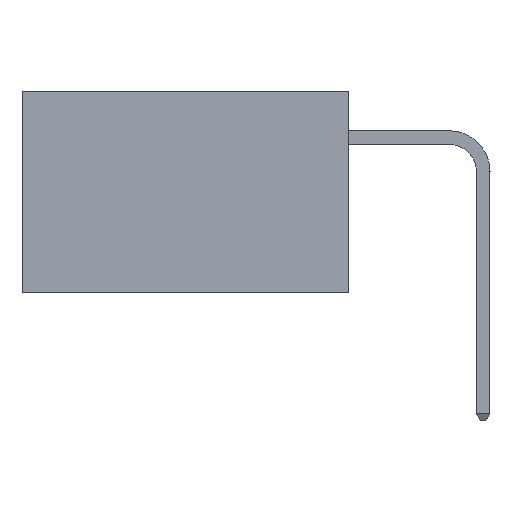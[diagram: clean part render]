
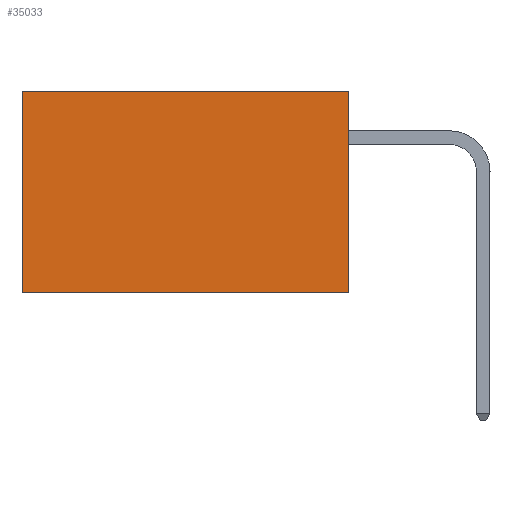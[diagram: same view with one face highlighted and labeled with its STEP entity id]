
A CAD part, left-side view. The second image highlights one B-rep face of the part: STEP entity #35033.
In plain terms, the highlighted planar face has unit normal (-1, 0, 0).
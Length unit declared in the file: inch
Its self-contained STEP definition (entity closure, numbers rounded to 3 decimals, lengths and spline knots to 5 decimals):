
#1095 = DIRECTION ( 'NONE',  ( 0., 1., 0. ) ) ;
#2598 = VERTEX_POINT ( 'NONE', #11360 ) ;
#3098 = CARTESIAN_POINT ( 'NONE',  ( 0.2875, 0., 0. ) ) ;
#3789 = CARTESIAN_POINT ( 'NONE',  ( 0.2875, 0., 0. ) ) ;
#5382 = VERTEX_POINT ( 'NONE', #20725 ) ;
#5522 = DIRECTION ( 'NONE',  ( 0., 0., -1. ) ) ;
#6307 = VERTEX_POINT ( 'NONE', #31010 ) ;
#6369 = ORIENTED_EDGE ( 'NONE', *, *, #20440, .F. ) ;
#6373 = DIRECTION ( 'NONE',  ( 0., 0., -1. ) ) ;
#7091 = EDGE_CURVE ( 'NONE', #6307, #5382, #21575, .T. ) ;
#8061 = LINE ( 'NONE', #3789, #22695 ) ;
#9188 = VECTOR ( 'NONE', #1095, 39.37008 ) ;
#11254 = DIRECTION ( 'NONE',  ( 0., 1., 0. ) ) ;
#11360 = CARTESIAN_POINT ( 'NONE',  ( 0.2875, 0.6, -0.37 ) ) ;
#11615 = EDGE_CURVE ( 'NONE', #14372, #2598, #17015, .T. ) ;
#14372 = VERTEX_POINT ( 'NONE', #28312 ) ;
#17015 = LINE ( 'NONE', #33896, #9188 ) ;
#17180 = CARTESIAN_POINT ( 'NONE',  ( 0.2875, 0., 0. ) ) ;
#18517 = ORIENTED_EDGE ( 'NONE', *, *, #35726, .T. ) ;
#18972 = LINE ( 'NONE', #23846, #35971 ) ;
#20125 = PLANE ( 'NONE',  #27266 ) ;
#20440 = EDGE_CURVE ( 'NONE', #6307, #14372, #8061, .T. ) ;
#20669 = VECTOR ( 'NONE', #11254, 39.37008 ) ;
#20725 = CARTESIAN_POINT ( 'NONE',  ( 0.2875, 0.6, 0. ) ) ;
#21575 = LINE ( 'NONE', #3098, #20669 ) ;
#22695 = VECTOR ( 'NONE', #35477, 39.37008 ) ;
#23015 = DIRECTION ( 'NONE',  ( 1., 0., 0. ) ) ;
#23846 = CARTESIAN_POINT ( 'NONE',  ( 0.2875, 0.6, 0. ) ) ;
#24268 = ORIENTED_EDGE ( 'NONE', *, *, #11615, .F. ) ;
#27266 = AXIS2_PLACEMENT_3D ( 'NONE', #17180, #23015, #5522 ) ;
#28312 = CARTESIAN_POINT ( 'NONE',  ( 0.2875, 0., -0.37 ) ) ;
#28890 = FACE_OUTER_BOUND ( 'NONE', #35016, .T. ) ;
#29421 = ORIENTED_EDGE ( 'NONE', *, *, #7091, .T. ) ;
#31010 = CARTESIAN_POINT ( 'NONE',  ( 0.2875, 0., 0. ) ) ;
#33896 = CARTESIAN_POINT ( 'NONE',  ( 0.2875, 0., -0.37 ) ) ;
#35016 = EDGE_LOOP ( 'NONE', ( #18517, #24268, #6369, #29421 ) ) ;
#35033 = ADVANCED_FACE ( 'NONE', ( #28890 ), #20125, .F. ) ;
#35477 = DIRECTION ( 'NONE',  ( 0., 0., -1. ) ) ;
#35726 = EDGE_CURVE ( 'NONE', #5382, #2598, #18972, .T. ) ;
#35971 = VECTOR ( 'NONE', #6373, 39.37008 ) ;
